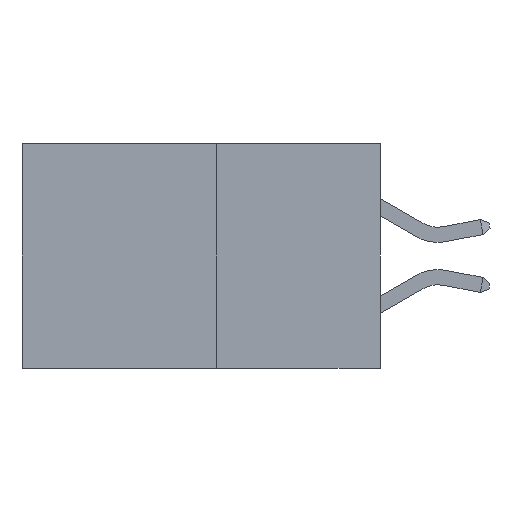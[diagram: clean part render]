
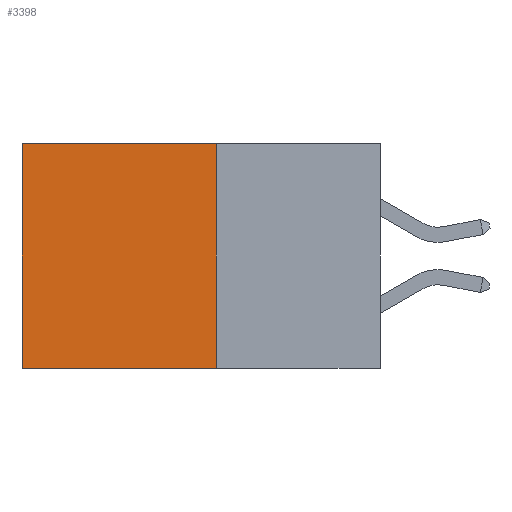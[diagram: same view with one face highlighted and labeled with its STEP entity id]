
A CAD part, left-side view. The second image highlights one B-rep face of the part: STEP entity #3398.
In plain terms, the highlighted planar face has unit normal (-1, 0, 0).
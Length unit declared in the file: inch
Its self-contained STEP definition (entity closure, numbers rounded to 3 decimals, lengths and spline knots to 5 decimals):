
#248 = EDGE_CURVE ( 'NONE', #2606, #2894, #1451, .T. ) ;
#932 = EDGE_CURVE ( 'NONE', #2606, #5118, #5180, .T. ) ;
#1162 = ORIENTED_EDGE ( 'NONE', *, *, #5210, .F. ) ;
#1451 = LINE ( 'NONE', #2786, #6944 ) ;
#1744 = CARTESIAN_POINT ( 'NONE',  ( 0.277, 0.59, -0.37 ) ) ;
#2402 = CARTESIAN_POINT ( 'NONE',  ( 0.277, 0.27, -0.37 ) ) ;
#2461 = DIRECTION ( 'NONE',  ( 0., 0., -1. ) ) ;
#2606 = VERTEX_POINT ( 'NONE', #7370 ) ;
#2656 = CARTESIAN_POINT ( 'NONE',  ( 0.277, 0.27, -0.37 ) ) ;
#2786 = CARTESIAN_POINT ( 'NONE',  ( 0.277, 0.27, -0.37 ) ) ;
#2833 = EDGE_LOOP ( 'NONE', ( #4341, #1162, #3784, #3340 ) ) ;
#2894 = VERTEX_POINT ( 'NONE', #8460 ) ;
#2904 = LINE ( 'NONE', #3118, #6274 ) ;
#3118 = CARTESIAN_POINT ( 'NONE',  ( 0.277, 0.59, -0.37 ) ) ;
#3340 = ORIENTED_EDGE ( 'NONE', *, *, #932, .T. ) ;
#3398 = ADVANCED_FACE ( 'NONE', ( #5839 ), #8114, .F. ) ;
#3501 = DIRECTION ( 'NONE',  ( 0., 0., -1. ) ) ;
#3695 = DIRECTION ( 'NONE',  ( 0., 0., -1. ) ) ;
#3754 = EDGE_CURVE ( 'NONE', #5118, #4538, #2904, .T. ) ;
#3784 = ORIENTED_EDGE ( 'NONE', *, *, #248, .F. ) ;
#3905 = CARTESIAN_POINT ( 'NONE',  ( 0.277, 0.59, 0. ) ) ;
#4341 = ORIENTED_EDGE ( 'NONE', *, *, #3754, .T. ) ;
#4538 = VERTEX_POINT ( 'NONE', #1744 ) ;
#4879 = VECTOR ( 'NONE', #6856, 39.37008 ) ;
#4959 = VECTOR ( 'NONE', #8945, 39.37008 ) ;
#5118 = VERTEX_POINT ( 'NONE', #3905 ) ;
#5180 = LINE ( 'NONE', #7793, #4959 ) ;
#5210 = EDGE_CURVE ( 'NONE', #2894, #4538, #6754, .T. ) ;
#5839 = FACE_OUTER_BOUND ( 'NONE', #2833, .T. ) ;
#5908 = AXIS2_PLACEMENT_3D ( 'NONE', #2402, #7710, #2461 ) ;
#6274 = VECTOR ( 'NONE', #3501, 39.37008 ) ;
#6754 = LINE ( 'NONE', #2656, #4879 ) ;
#6856 = DIRECTION ( 'NONE',  ( 0., 1., 0. ) ) ;
#6944 = VECTOR ( 'NONE', #3695, 39.37008 ) ;
#7370 = CARTESIAN_POINT ( 'NONE',  ( 0.277, 0.27, 0. ) ) ;
#7710 = DIRECTION ( 'NONE',  ( 1., 0., 0. ) ) ;
#7793 = CARTESIAN_POINT ( 'NONE',  ( 0.277, 0.27, 0. ) ) ;
#8114 = PLANE ( 'NONE',  #5908 ) ;
#8460 = CARTESIAN_POINT ( 'NONE',  ( 0.277, 0.27, -0.37 ) ) ;
#8945 = DIRECTION ( 'NONE',  ( 0., 1., 0. ) ) ;
